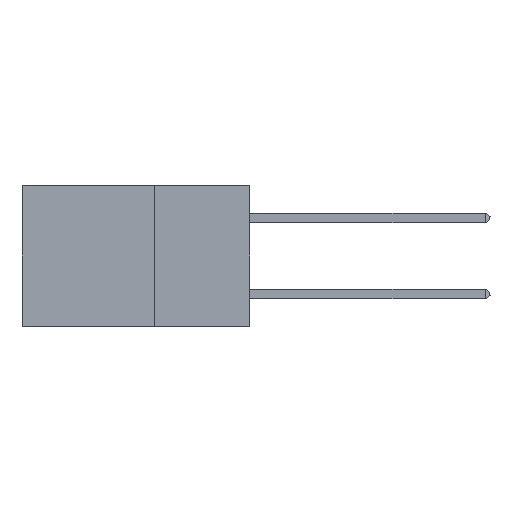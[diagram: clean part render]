
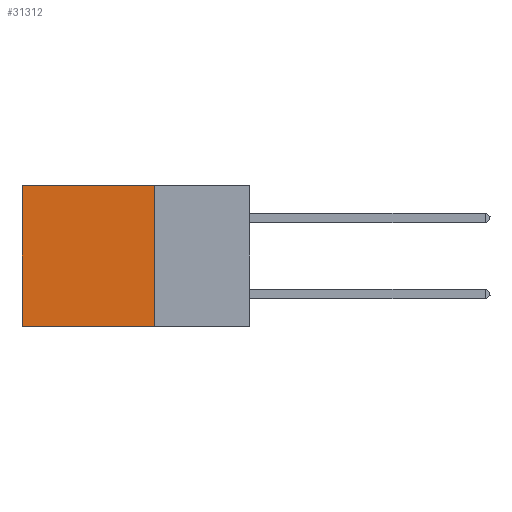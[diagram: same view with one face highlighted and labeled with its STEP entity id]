
A CAD part, left-side view. The second image highlights one B-rep face of the part: STEP entity #31312.
In plain terms, the highlighted planar face has unit normal (-1, 0, 0).
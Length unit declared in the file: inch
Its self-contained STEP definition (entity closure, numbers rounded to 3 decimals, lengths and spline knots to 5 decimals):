
#126 = PLANE ( 'NONE',  #9671 ) ;
#1477 = ORIENTED_EDGE ( 'NONE', *, *, #9042, .F. ) ;
#1501 = DIRECTION ( 'NONE',  ( 0., 1., 0. ) ) ;
#4767 = CARTESIAN_POINT ( 'NONE',  ( 0.2875, 0.6, 0. ) ) ;
#5635 = VECTOR ( 'NONE', #16982, 39.37008 ) ;
#5872 = VERTEX_POINT ( 'NONE', #8607 ) ;
#6116 = ORIENTED_EDGE ( 'NONE', *, *, #43308, .T. ) ;
#8048 = VERTEX_POINT ( 'NONE', #26837 ) ;
#8607 = CARTESIAN_POINT ( 'NONE',  ( 0.2875, 0.25, -0.37 ) ) ;
#9042 = EDGE_CURVE ( 'NONE', #5872, #17011, #12291, .T. ) ;
#9211 = LINE ( 'NONE', #40709, #26268 ) ;
#9671 = AXIS2_PLACEMENT_3D ( 'NONE', #27246, #34214, #40883 ) ;
#9992 = ORIENTED_EDGE ( 'NONE', *, *, #14956, .T. ) ;
#12291 = LINE ( 'NONE', #14763, #43160 ) ;
#13702 = CARTESIAN_POINT ( 'NONE',  ( 0.2875, 0.25, 0. ) ) ;
#14595 = VERTEX_POINT ( 'NONE', #4767 ) ;
#14763 = CARTESIAN_POINT ( 'NONE',  ( 0.2875, 0.25, -0.37 ) ) ;
#14956 = EDGE_CURVE ( 'NONE', #14595, #17011, #35858, .T. ) ;
#16982 = DIRECTION ( 'NONE',  ( 0., 1., 0. ) ) ;
#17011 = VERTEX_POINT ( 'NONE', #25402 ) ;
#23923 = DIRECTION ( 'NONE',  ( 0., 0., -1. ) ) ;
#24639 = ORIENTED_EDGE ( 'NONE', *, *, #39066, .F. ) ;
#24790 = EDGE_LOOP ( 'NONE', ( #9992, #1477, #24639, #6116 ) ) ;
#25402 = CARTESIAN_POINT ( 'NONE',  ( 0.2875, 0.6, -0.37 ) ) ;
#26268 = VECTOR ( 'NONE', #23923, 39.37008 ) ;
#26837 = CARTESIAN_POINT ( 'NONE',  ( 0.2875, 0.25, 0. ) ) ;
#27023 = FACE_OUTER_BOUND ( 'NONE', #24790, .T. ) ;
#27246 = CARTESIAN_POINT ( 'NONE',  ( 0.2875, 0.25, 0. ) ) ;
#31312 = ADVANCED_FACE ( 'NONE', ( #27023 ), #126, .F. ) ;
#34214 = DIRECTION ( 'NONE',  ( 1., 0., 0. ) ) ;
#34375 = CARTESIAN_POINT ( 'NONE',  ( 0.2875, 0.6, 0. ) ) ;
#35858 = LINE ( 'NONE', #34375, #41713 ) ;
#37921 = DIRECTION ( 'NONE',  ( 0., 0., -1. ) ) ;
#39066 = EDGE_CURVE ( 'NONE', #8048, #5872, #9211, .T. ) ;
#40709 = CARTESIAN_POINT ( 'NONE',  ( 0.2875, 0.25, 0. ) ) ;
#40883 = DIRECTION ( 'NONE',  ( 0., 0., -1. ) ) ;
#41713 = VECTOR ( 'NONE', #37921, 39.37008 ) ;
#41828 = LINE ( 'NONE', #13702, #5635 ) ;
#43160 = VECTOR ( 'NONE', #1501, 39.37008 ) ;
#43308 = EDGE_CURVE ( 'NONE', #8048, #14595, #41828, .T. ) ;
